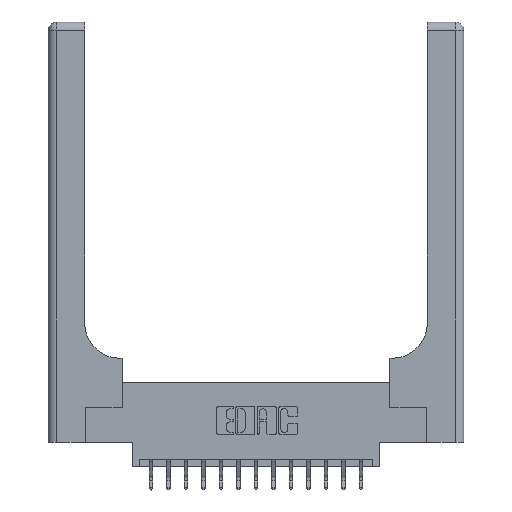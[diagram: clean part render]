
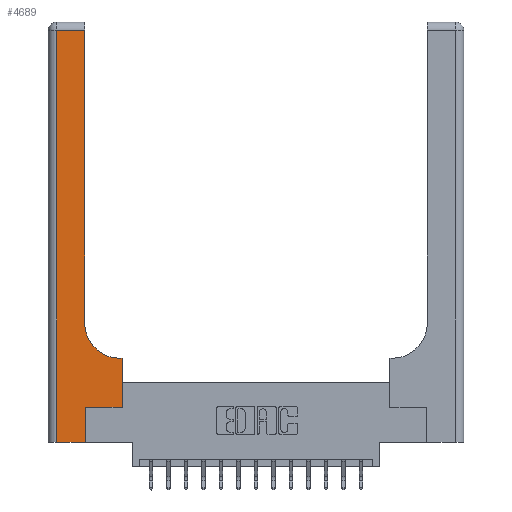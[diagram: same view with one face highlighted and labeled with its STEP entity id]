
A CAD part, top view. The second image highlights one B-rep face of the part: STEP entity #4689.
In plain terms, the highlighted planar face has unit normal (0, 0, 1).
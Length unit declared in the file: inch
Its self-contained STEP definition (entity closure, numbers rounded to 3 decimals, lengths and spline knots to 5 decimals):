
#131 = VERTEX_POINT ( 'NONE', #5279 ) ;
#374 = ORIENTED_EDGE ( 'NONE', *, *, #1832, .T. ) ;
#632 = VERTEX_POINT ( 'NONE', #2284 ) ;
#639 = ORIENTED_EDGE ( 'NONE', *, *, #14736, .T. ) ;
#664 = CARTESIAN_POINT ( 'NONE',  ( 0.528, 0.25, 0.37 ) ) ;
#833 = CARTESIAN_POINT ( 'NONE',  ( 0.265, 0.25, 0.37 ) ) ;
#1136 = VECTOR ( 'NONE', #9004, 39.37008 ) ;
#1574 = ORIENTED_EDGE ( 'NONE', *, *, #1966, .T. ) ;
#1651 = CIRCLE ( 'NONE', #13168, 0.25 ) ;
#1790 = LINE ( 'NONE', #17373, #5113 ) ;
#1832 = EDGE_CURVE ( 'NONE', #5994, #12141, #1790, .T. ) ;
#1966 = EDGE_CURVE ( 'NONE', #131, #4151, #7041, .T. ) ;
#1992 = CARTESIAN_POINT ( 'NONE',  ( 0.51, 0.6, 0.37 ) ) ;
#2284 = CARTESIAN_POINT ( 'NONE',  ( 0.26, 2.94, 0.37 ) ) ;
#2372 = VECTOR ( 'NONE', #8799, 39.37008 ) ;
#2374 = EDGE_LOOP ( 'NONE', ( #13585, #13860, #639, #374, #17772, #15104, #8051, #1574, #8429 ) ) ;
#2383 = VERTEX_POINT ( 'NONE', #2539 ) ;
#2468 = EDGE_CURVE ( 'NONE', #632, #16534, #14962, .T. ) ;
#2539 = CARTESIAN_POINT ( 'NONE',  ( 0.26, 0.85, 0.37 ) ) ;
#3713 = LINE ( 'NONE', #14107, #11075 ) ;
#4151 = VERTEX_POINT ( 'NONE', #1992 ) ;
#4347 = VECTOR ( 'NONE', #11043, 39.37008 ) ;
#4689 = ADVANCED_FACE ( 'NONE', ( #4736 ), #13024, .F. ) ;
#4736 = FACE_OUTER_BOUND ( 'NONE', #2374, .T. ) ;
#4753 = DIRECTION ( 'NONE',  ( 0., 0., -1. ) ) ;
#4925 = EDGE_CURVE ( 'NONE', #2383, #632, #12711, .T. ) ;
#5113 = VECTOR ( 'NONE', #7714, 39.37008 ) ;
#5279 = CARTESIAN_POINT ( 'NONE',  ( 0.528, 0.6, 0.37 ) ) ;
#5842 = DIRECTION ( 'NONE',  ( 0., 1., 0. ) ) ;
#5953 = DIRECTION ( 'NONE',  ( 0., 0., -1. ) ) ;
#5994 = VERTEX_POINT ( 'NONE', #17775 ) ;
#6817 = EDGE_CURVE ( 'NONE', #7214, #131, #12202, .T. ) ;
#7041 = LINE ( 'NONE', #7950, #13968 ) ;
#7214 = VERTEX_POINT ( 'NONE', #14323 ) ;
#7231 = DIRECTION ( 'NONE',  ( 1., 0., 0. ) ) ;
#7405 = CARTESIAN_POINT ( 'NONE',  ( 0., 3., 0.37 ) ) ;
#7556 = VECTOR ( 'NONE', #7231, 39.37008 ) ;
#7714 = DIRECTION ( 'NONE',  ( 1., 0., 0. ) ) ;
#7950 = CARTESIAN_POINT ( 'NONE',  ( 0.26, 0.6, 0.37 ) ) ;
#8051 = ORIENTED_EDGE ( 'NONE', *, *, #6817, .T. ) ;
#8096 = VERTEX_POINT ( 'NONE', #833 ) ;
#8429 = ORIENTED_EDGE ( 'NONE', *, *, #9629, .T. ) ;
#8799 = DIRECTION ( 'NONE',  ( 0., -1., 0. ) ) ;
#9004 = DIRECTION ( 'NONE',  ( 0., 1., 0. ) ) ;
#9629 = EDGE_CURVE ( 'NONE', #4151, #2383, #1651, .T. ) ;
#10266 = EDGE_CURVE ( 'NONE', #8096, #7214, #11218, .T. ) ;
#10632 = CARTESIAN_POINT ( 'NONE',  ( 0.06, 2.94, 0.37 ) ) ;
#11043 = DIRECTION ( 'NONE',  ( -1., 0., 0. ) ) ;
#11075 = VECTOR ( 'NONE', #5842, 39.37008 ) ;
#11218 = LINE ( 'NONE', #14137, #7556 ) ;
#11811 = AXIS2_PLACEMENT_3D ( 'NONE', #7405, #4753, #14437 ) ;
#12141 = VERTEX_POINT ( 'NONE', #13562 ) ;
#12202 = LINE ( 'NONE', #664, #1136 ) ;
#12711 = LINE ( 'NONE', #15145, #15535 ) ;
#13024 = PLANE ( 'NONE',  #11811 ) ;
#13168 = AXIS2_PLACEMENT_3D ( 'NONE', #14218, #5953, #15593 ) ;
#13513 = DIRECTION ( 'NONE',  ( 0., 1., 0. ) ) ;
#13562 = CARTESIAN_POINT ( 'NONE',  ( 0.265, 0., 0.37 ) ) ;
#13585 = ORIENTED_EDGE ( 'NONE', *, *, #4925, .T. ) ;
#13860 = ORIENTED_EDGE ( 'NONE', *, *, #2468, .T. ) ;
#13968 = VECTOR ( 'NONE', #16253, 39.37008 ) ;
#14107 = CARTESIAN_POINT ( 'NONE',  ( 0.265, 0., 0.37 ) ) ;
#14137 = CARTESIAN_POINT ( 'NONE',  ( 0.265, 0.25, 0.37 ) ) ;
#14218 = CARTESIAN_POINT ( 'NONE',  ( 0.51, 0.85, 0.37 ) ) ;
#14323 = CARTESIAN_POINT ( 'NONE',  ( 0.528, 0.25, 0.37 ) ) ;
#14327 = CARTESIAN_POINT ( 'NONE',  ( 0.06, 3., 0.37 ) ) ;
#14437 = DIRECTION ( 'NONE',  ( -1., 0., 0. ) ) ;
#14736 = EDGE_CURVE ( 'NONE', #16534, #5994, #17109, .T. ) ;
#14962 = LINE ( 'NONE', #17911, #4347 ) ;
#15104 = ORIENTED_EDGE ( 'NONE', *, *, #10266, .T. ) ;
#15145 = CARTESIAN_POINT ( 'NONE',  ( 0.26, 3., 0.37 ) ) ;
#15535 = VECTOR ( 'NONE', #13513, 39.37008 ) ;
#15593 = DIRECTION ( 'NONE',  ( 1., 0., 0. ) ) ;
#16253 = DIRECTION ( 'NONE',  ( -1., 0., 0. ) ) ;
#16307 = EDGE_CURVE ( 'NONE', #12141, #8096, #3713, .T. ) ;
#16534 = VERTEX_POINT ( 'NONE', #10632 ) ;
#17109 = LINE ( 'NONE', #14327, #2372 ) ;
#17373 = CARTESIAN_POINT ( 'NONE',  ( 0., 0., 0.37 ) ) ;
#17772 = ORIENTED_EDGE ( 'NONE', *, *, #16307, .T. ) ;
#17775 = CARTESIAN_POINT ( 'NONE',  ( 0.06, 0., 0.37 ) ) ;
#17911 = CARTESIAN_POINT ( 'NONE',  ( 0., 2.94, 0.37 ) ) ;
